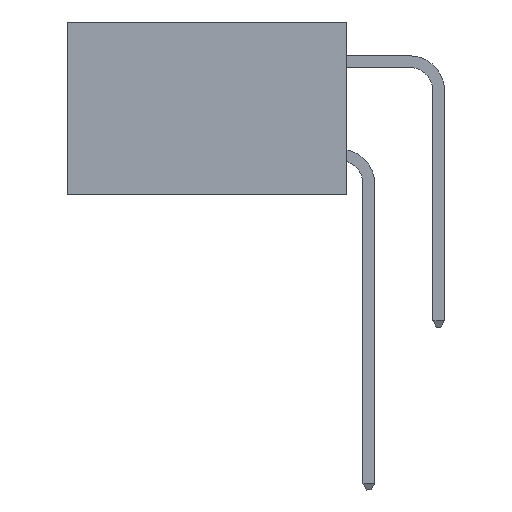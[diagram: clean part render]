
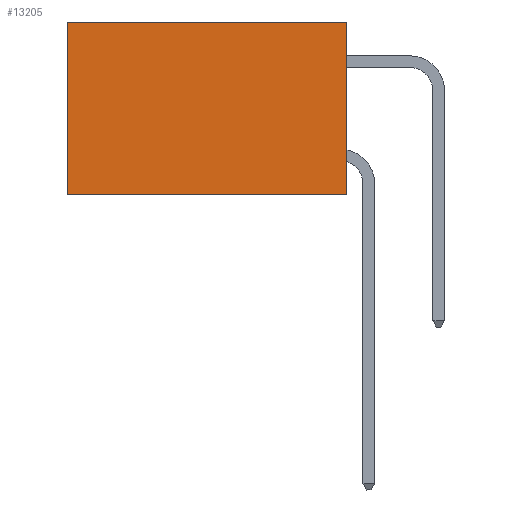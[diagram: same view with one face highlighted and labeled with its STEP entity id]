
A CAD part, left-side view. The second image highlights one B-rep face of the part: STEP entity #13205.
In plain terms, the highlighted planar face has unit normal (-1, 0, 0).
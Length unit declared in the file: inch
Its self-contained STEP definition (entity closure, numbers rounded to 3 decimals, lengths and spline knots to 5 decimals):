
#1604 = VECTOR ( 'NONE', #17331, 39.37008 ) ;
#2882 = VECTOR ( 'NONE', #11833, 39.37008 ) ;
#3391 = DIRECTION ( 'NONE',  ( 0., 0., -1. ) ) ;
#3585 = LINE ( 'NONE', #3688, #20618 ) ;
#3688 = CARTESIAN_POINT ( 'NONE',  ( 0.2875, 0.6, 0. ) ) ;
#3710 = CARTESIAN_POINT ( 'NONE',  ( 0.2875, 0., 0. ) ) ;
#4963 = EDGE_CURVE ( 'NONE', #7937, #7910, #5434, .T. ) ;
#5090 = FACE_OUTER_BOUND ( 'NONE', #17402, .T. ) ;
#5166 = VERTEX_POINT ( 'NONE', #5798 ) ;
#5434 = LINE ( 'NONE', #13326, #18477 ) ;
#5798 = CARTESIAN_POINT ( 'NONE',  ( 0.2875, 0.6, 0. ) ) ;
#7013 = VERTEX_POINT ( 'NONE', #8690 ) ;
#7413 = LINE ( 'NONE', #18615, #2882 ) ;
#7641 = ORIENTED_EDGE ( 'NONE', *, *, #14002, .T. ) ;
#7910 = VERTEX_POINT ( 'NONE', #18105 ) ;
#7937 = VERTEX_POINT ( 'NONE', #19887 ) ;
#8690 = CARTESIAN_POINT ( 'NONE',  ( 0.2875, 0.6, -0.37 ) ) ;
#9905 = DIRECTION ( 'NONE',  ( 0., 0., -1. ) ) ;
#10148 = CARTESIAN_POINT ( 'NONE',  ( 0.2875, 0., 0. ) ) ;
#10313 = ORIENTED_EDGE ( 'NONE', *, *, #14621, .F. ) ;
#11833 = DIRECTION ( 'NONE',  ( 0., 1., 0. ) ) ;
#11865 = PLANE ( 'NONE',  #19628 ) ;
#13137 = ORIENTED_EDGE ( 'NONE', *, *, #4963, .F. ) ;
#13205 = ADVANCED_FACE ( 'NONE', ( #5090 ), #11865, .F. ) ;
#13326 = CARTESIAN_POINT ( 'NONE',  ( 0.2875, 0., 0. ) ) ;
#13572 = DIRECTION ( 'NONE',  ( 1., 0., 0. ) ) ;
#14002 = EDGE_CURVE ( 'NONE', #7937, #5166, #19679, .T. ) ;
#14621 = EDGE_CURVE ( 'NONE', #7910, #7013, #7413, .T. ) ;
#15588 = DIRECTION ( 'NONE',  ( 0., 0., -1. ) ) ;
#17331 = DIRECTION ( 'NONE',  ( 0., 1., 0. ) ) ;
#17402 = EDGE_LOOP ( 'NONE', ( #18535, #10313, #13137, #7641 ) ) ;
#18105 = CARTESIAN_POINT ( 'NONE',  ( 0.2875, 0., -0.37 ) ) ;
#18477 = VECTOR ( 'NONE', #9905, 39.37008 ) ;
#18535 = ORIENTED_EDGE ( 'NONE', *, *, #21315, .T. ) ;
#18615 = CARTESIAN_POINT ( 'NONE',  ( 0.2875, 0., -0.37 ) ) ;
#19628 = AXIS2_PLACEMENT_3D ( 'NONE', #10148, #13572, #3391 ) ;
#19679 = LINE ( 'NONE', #3710, #1604 ) ;
#19887 = CARTESIAN_POINT ( 'NONE',  ( 0.2875, 0., 0. ) ) ;
#20618 = VECTOR ( 'NONE', #15588, 39.37008 ) ;
#21315 = EDGE_CURVE ( 'NONE', #5166, #7013, #3585, .T. ) ;
